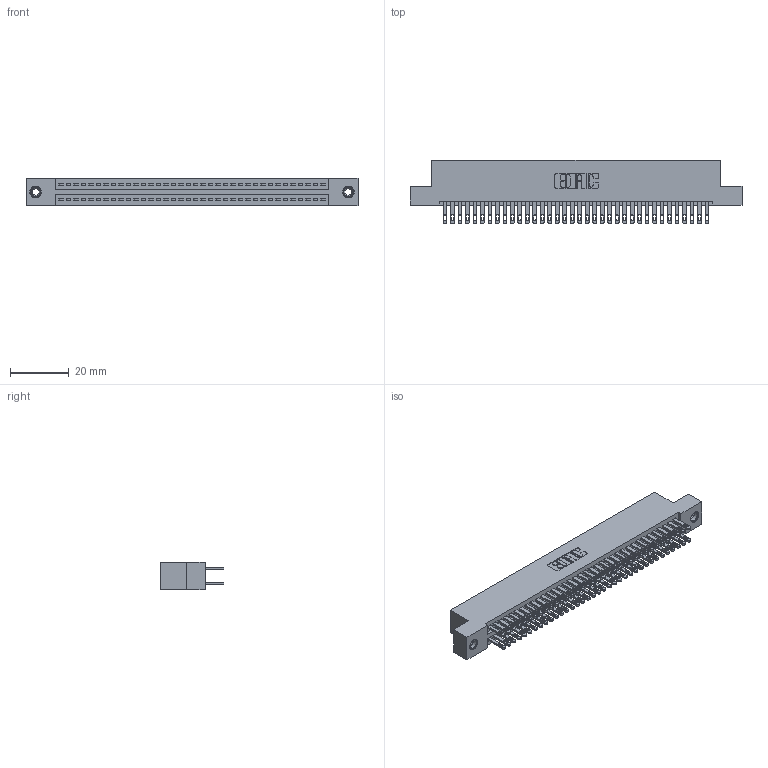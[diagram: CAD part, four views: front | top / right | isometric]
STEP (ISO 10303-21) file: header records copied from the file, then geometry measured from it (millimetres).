
FILE_DESCRIPTION (( 'STEP AP203' ), '1' );
FILE_NAME ('345-072-500-208.STEP', '2018-10-01T17:24:51', ( '' ), ( '' ), 'SwSTEP 2.0', 'SolidWorks 2016', '' );
FILE_SCHEMA (( 'CONFIG_CONTROL_DESIGN' ));
Length unit declared in the file: inch
Products named in the file (4): 345-292-001_345-293-100; 345-072-500-208; 345-250-001_345-250-003-102; 345 Part_Flush Mounting Lugs - 0.156 Dia-TI
Assembly tree (75 placements, depth 2):
  345-072-500-208
    345 Part_Flush Mounting Lugs - 0.156 Dia-TI
    345-292-001_345-293-100  x72
    345-250-001_345-250-003-102  x2
Bounding box: 112.65 x 21.51 x 9.4 mm (x, y, z)
Volume: 11100.6 mm3; surface area: 17040.2 mm2
Topology: 75 solids, 75 shells, 3498 faces, 10629 edges, 7078 vertices
Faces by surface type: plane 2056, cylinder 1426, cone 12, torus 4
Entity records: 30170 total; most frequent: CARTESIAN_POINT 5043, ORIENTED_EDGE 4970, DIRECTION 4483, EDGE_CURVE 2485, LINE 2185, VECTOR 2185, VERTEX_POINT 1652, AXIS2_PLACEMENT_3D 1149
